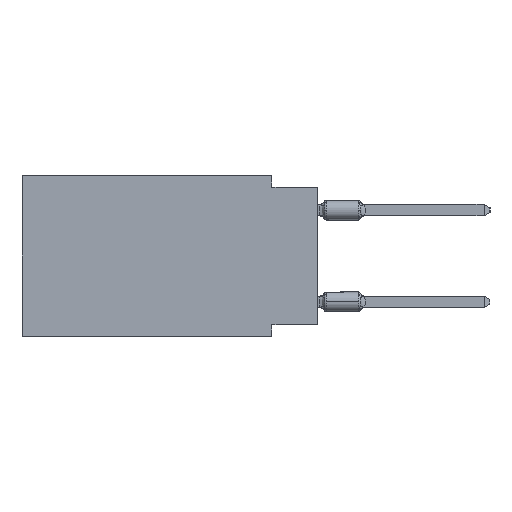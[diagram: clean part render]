
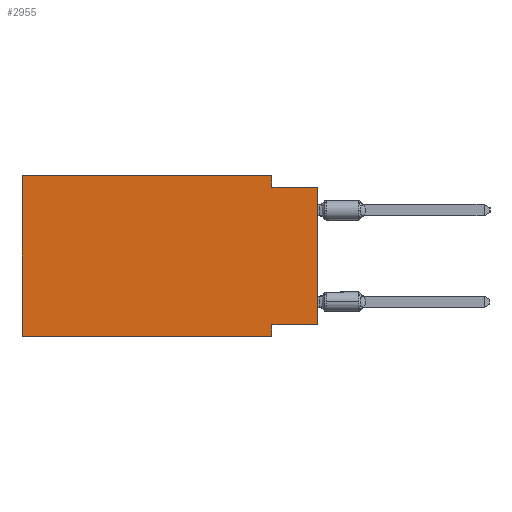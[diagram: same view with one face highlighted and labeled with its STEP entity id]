
A CAD part, left-side view. The second image highlights one B-rep face of the part: STEP entity #2955.
In plain terms, the highlighted planar face has unit normal (-1, 0, 0).
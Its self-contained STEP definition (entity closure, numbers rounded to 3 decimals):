
#289 = VERTEX_POINT ( 'NONE', #417 ) ;
#417 = CARTESIAN_POINT ( 'NONE',  ( 0., 0., -8.255 ) ) ;
#591 = ORIENTED_EDGE ( 'NONE', *, *, #42052, .F. ) ;
#1890 = DIRECTION ( 'NONE',  ( 0., 0., -1. ) ) ;
#2000 = LINE ( 'NONE', #41894, #36908 ) ;
#2955 = ADVANCED_FACE ( 'NONE', ( #42051 ), #25352, .F. ) ;
#4372 = CARTESIAN_POINT ( 'NONE',  ( 0., 0., 0. ) ) ;
#6498 = VERTEX_POINT ( 'NONE', #29611 ) ;
#6722 = DIRECTION ( 'NONE',  ( 0., 1., 0. ) ) ;
#7528 = EDGE_CURVE ( 'NONE', #37742, #44291, #27571, .T. ) ;
#9999 = DIRECTION ( 'NONE',  ( 0., -1., 0. ) ) ;
#10892 = LINE ( 'NONE', #34867, #25783 ) ;
#12246 = CARTESIAN_POINT ( 'NONE',  ( 0., 2.54, -8.255 ) ) ;
#12504 = VERTEX_POINT ( 'NONE', #12246 ) ;
#12685 = VECTOR ( 'NONE', #44014, 1000. ) ;
#13344 = ORIENTED_EDGE ( 'NONE', *, *, #15478, .T. ) ;
#13914 = LINE ( 'NONE', #45729, #41762 ) ;
#15478 = EDGE_CURVE ( 'NONE', #37742, #6498, #16591, .T. ) ;
#15603 = CARTESIAN_POINT ( 'NONE',  ( 0., 16.383, 0. ) ) ;
#16545 = VECTOR ( 'NONE', #26898, 1000. ) ;
#16591 = LINE ( 'NONE', #17118, #41474 ) ;
#17118 = CARTESIAN_POINT ( 'NONE',  ( 0., 16.383, -8.89 ) ) ;
#22427 = VECTOR ( 'NONE', #37756, 1000. ) ;
#22737 = LINE ( 'NONE', #38655, #16545 ) ;
#22767 = EDGE_CURVE ( 'NONE', #26003, #38009, #2000, .T. ) ;
#23026 = VERTEX_POINT ( 'NONE', #40792 ) ;
#24260 = EDGE_LOOP ( 'NONE', ( #49733, #39748, #591, #43212, #32314, #13344, #42427, #32473 ) ) ;
#25352 = PLANE ( 'NONE',  #28959 ) ;
#25595 = DIRECTION ( 'NONE',  ( 1., 0., 0. ) ) ;
#25783 = VECTOR ( 'NONE', #6722, 1000. ) ;
#26003 = VERTEX_POINT ( 'NONE', #42426 ) ;
#26898 = DIRECTION ( 'NONE',  ( 0., 0., -1. ) ) ;
#27571 = LINE ( 'NONE', #15603, #12685 ) ;
#28326 = LINE ( 'NONE', #4372, #47382 ) ;
#28959 = AXIS2_PLACEMENT_3D ( 'NONE', #37085, #25595, #1890 ) ;
#29611 = CARTESIAN_POINT ( 'NONE',  ( 0., 2.54, -8.89 ) ) ;
#29651 = LINE ( 'NONE', #45587, #22427 ) ;
#30875 = CARTESIAN_POINT ( 'NONE',  ( 0., 0., -0.635 ) ) ;
#32314 = ORIENTED_EDGE ( 'NONE', *, *, #7528, .F. ) ;
#32473 = ORIENTED_EDGE ( 'NONE', *, *, #42859, .F. ) ;
#34867 = CARTESIAN_POINT ( 'NONE',  ( 0., 0., -8.255 ) ) ;
#36908 = VECTOR ( 'NONE', #42400, 1000. ) ;
#37085 = CARTESIAN_POINT ( 'NONE',  ( 0., 16.383, 0. ) ) ;
#37742 = VERTEX_POINT ( 'NONE', #43230 ) ;
#37756 = DIRECTION ( 'NONE',  ( 0., 0., -1. ) ) ;
#38009 = VERTEX_POINT ( 'NONE', #30875 ) ;
#38655 = CARTESIAN_POINT ( 'NONE',  ( 0., 2.54, 0. ) ) ;
#39748 = ORIENTED_EDGE ( 'NONE', *, *, #22767, .F. ) ;
#40620 = EDGE_CURVE ( 'NONE', #289, #38009, #28326, .T. ) ;
#40792 = CARTESIAN_POINT ( 'NONE',  ( 0., 2.54, 0. ) ) ;
#41474 = VECTOR ( 'NONE', #44763, 1000. ) ;
#41762 = VECTOR ( 'NONE', #9999, 1000. ) ;
#41894 = CARTESIAN_POINT ( 'NONE',  ( 0., 0., -0.635 ) ) ;
#42051 = FACE_OUTER_BOUND ( 'NONE', #24260, .T. ) ;
#42052 = EDGE_CURVE ( 'NONE', #23026, #26003, #22737, .T. ) ;
#42400 = DIRECTION ( 'NONE',  ( 0., -1., 0. ) ) ;
#42426 = CARTESIAN_POINT ( 'NONE',  ( 0., 2.54, -0.635 ) ) ;
#42427 = ORIENTED_EDGE ( 'NONE', *, *, #42790, .F. ) ;
#42790 = EDGE_CURVE ( 'NONE', #12504, #6498, #29651, .T. ) ;
#42859 = EDGE_CURVE ( 'NONE', #289, #12504, #10892, .T. ) ;
#43212 = ORIENTED_EDGE ( 'NONE', *, *, #51148, .F. ) ;
#43230 = CARTESIAN_POINT ( 'NONE',  ( 0., 16.383, -8.89 ) ) ;
#43500 = DIRECTION ( 'NONE',  ( 0., 0., 1. ) ) ;
#44014 = DIRECTION ( 'NONE',  ( 0., 0., 1. ) ) ;
#44291 = VERTEX_POINT ( 'NONE', #45794 ) ;
#44763 = DIRECTION ( 'NONE',  ( 0., -1., 0. ) ) ;
#45587 = CARTESIAN_POINT ( 'NONE',  ( 0., 2.54, -8.89 ) ) ;
#45729 = CARTESIAN_POINT ( 'NONE',  ( 0., 16.383, 0. ) ) ;
#45794 = CARTESIAN_POINT ( 'NONE',  ( 0., 16.383, 0. ) ) ;
#47382 = VECTOR ( 'NONE', #43500, 1000. ) ;
#49733 = ORIENTED_EDGE ( 'NONE', *, *, #40620, .T. ) ;
#51148 = EDGE_CURVE ( 'NONE', #44291, #23026, #13914, .T. ) ;
